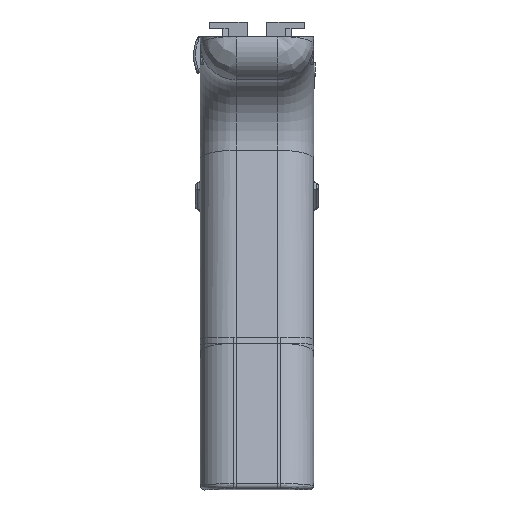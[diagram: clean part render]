
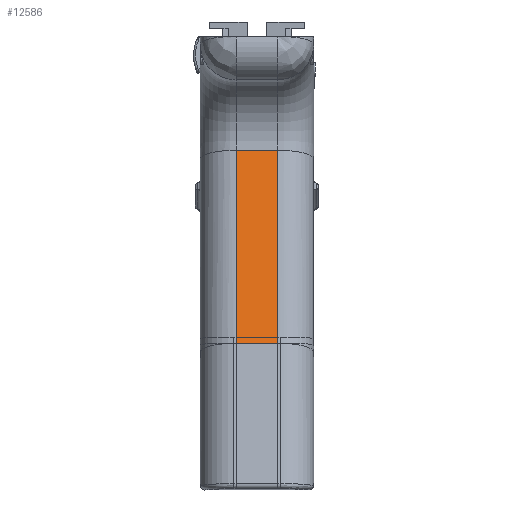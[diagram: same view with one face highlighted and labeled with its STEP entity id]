
A CAD part, front view. The second image highlights one B-rep face of the part: STEP entity #12586.
In plain terms, the highlighted face is planar.
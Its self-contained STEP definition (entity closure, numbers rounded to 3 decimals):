
#939=PLANE('',#13717);
#1499=FACE_OUTER_BOUND('',#2231,.T.);
#2231=EDGE_LOOP('',(#10684,#10685,#10686,#10687));
#3177=LINE('',#21345,#4323);
#3331=LINE('',#22190,#4477);
#3332=LINE('',#22193,#4478);
#3333=LINE('',#22194,#4479);
#4323=VECTOR('',#16072,10.);
#4477=VECTOR('',#16472,10.);
#4478=VECTOR('',#16475,10.);
#4479=VECTOR('',#16476,10.);
#5862=VERTEX_POINT('',#21341);
#5863=VERTEX_POINT('',#21343);
#5998=VERTEX_POINT('',#22168);
#6001=VERTEX_POINT('',#22192);
#7422=EDGE_CURVE('',#5862,#5863,#3177,.T.);
#7646=EDGE_CURVE('',#5862,#5998,#3331,.T.);
#7647=EDGE_CURVE('',#6001,#5863,#3332,.T.);
#7648=EDGE_CURVE('',#5998,#6001,#3333,.T.);
#10684=ORIENTED_EDGE('',*,*,#7647,.F.);
#10685=ORIENTED_EDGE('',*,*,#7648,.F.);
#10686=ORIENTED_EDGE('',*,*,#7646,.F.);
#10687=ORIENTED_EDGE('',*,*,#7422,.T.);
#12586=ADVANCED_FACE('',(#1499),#939,.T.);
#13717=AXIS2_PLACEMENT_3D('',#22191,#16473,#16474);
#16072=DIRECTION('',(0.,-0.249,0.969));
#16472=DIRECTION('',(-1.,0.,0.));
#16473=DIRECTION('center_axis',(0.,-0.969,
-0.249));
#16474=DIRECTION('ref_axis',(0.,-0.249,0.969));
#16475=DIRECTION('',(1.,0.,0.));
#16476=DIRECTION('',(0.,-0.249,0.969));
#21341=CARTESIAN_POINT('',(13.45,-71.634,19.877));
#21343=CARTESIAN_POINT('',(13.45,-83.628,66.536));
#21345=CARTESIAN_POINT('',(13.45,-83.554,66.245));
#22168=CARTESIAN_POINT('',(3.45,-71.634,19.877));
#22190=CARTESIAN_POINT('',(22.175,-71.634,19.877));
#22191=CARTESIAN_POINT('Origin',(22.175,-71.634,19.877));
#22192=CARTESIAN_POINT('',(3.45,-83.628,66.536));
#22193=CARTESIAN_POINT('',(22.175,-83.628,66.536));
#22194=CARTESIAN_POINT('',(3.45,-83.554,66.245));
